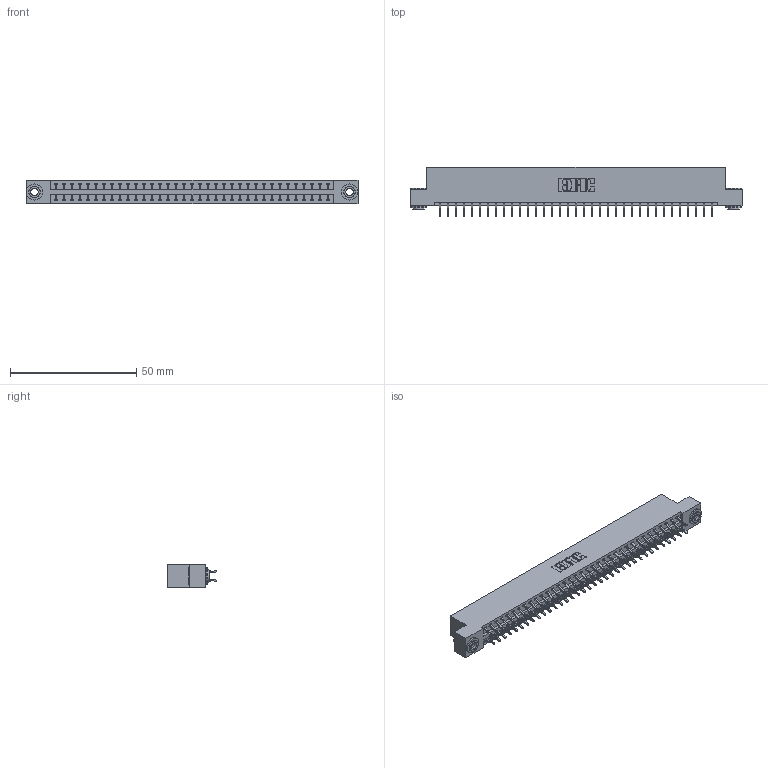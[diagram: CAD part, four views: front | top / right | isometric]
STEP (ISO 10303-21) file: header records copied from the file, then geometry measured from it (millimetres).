
FILE_DESCRIPTION (( 'STEP AP203' ), '1' );
FILE_NAME ('346-070-556-203.STEP', '2018-08-28T23:41:55', ( '' ), ( '' ), 'SwSTEP 2.0', 'SolidWorks 2016', '' );
FILE_SCHEMA (( 'CONFIG_CONTROL_DESIGN' ));
Length unit declared in the file: inch
Products named in the file (4): 345-292-001_556 Tail; 345-250-002_345-250-002-102; 346-070-556-203; 346 Part_Flush Mounting Lugs - 0.156 Dia-TH
Assembly tree (73 placements, depth 2):
  346-070-556-203
    346 Part_Flush Mounting Lugs - 0.156 Dia-TH
    345-292-001_556 Tail  x70
    345-250-002_345-250-002-102  x2
Bounding box: 131.7 x 19.57 x 9.4 mm (x, y, z)
Volume: 12804.5 mm3; surface area: 17639.8 mm2
Topology: 73 solids, 73 shells, 4220 faces, 12515 edges, 8246 vertices
Faces by surface type: plane 2816, cylinder 1396, cone 8
Entity records: 24654 total; most frequent: CARTESIAN_POINT 4063, ORIENTED_EDGE 3978, DIRECTION 3651, EDGE_CURVE 1989, LINE 1685, VECTOR 1685, VERTEX_POINT 1322, AXIS2_PLACEMENT_3D 983
